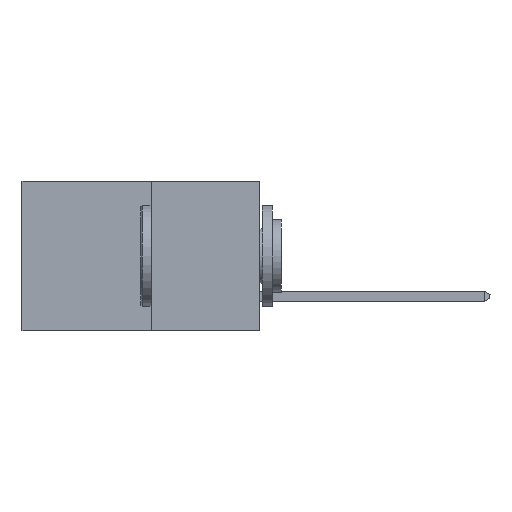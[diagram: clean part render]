
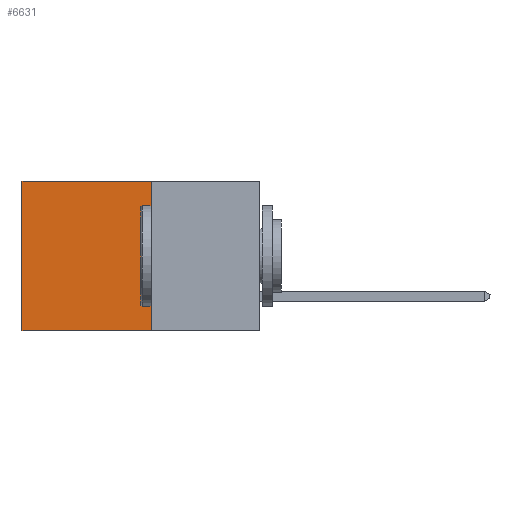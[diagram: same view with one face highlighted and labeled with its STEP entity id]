
A CAD part, left-side view. The second image highlights one B-rep face of the part: STEP entity #6631.
In plain terms, the highlighted planar face has unit normal (-1, 0, 0).
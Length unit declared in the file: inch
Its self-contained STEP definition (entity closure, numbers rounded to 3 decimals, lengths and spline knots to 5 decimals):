
#908 = EDGE_CURVE ( 'NONE', #919, #8544, #1760, .T. ) ;
#919 = VERTEX_POINT ( 'NONE', #2599 ) ;
#1028 = VERTEX_POINT ( 'NONE', #2394 ) ;
#1092 = EDGE_CURVE ( 'NONE', #4921, #1028, #3970, .T. ) ;
#1102 = ORIENTED_EDGE ( 'NONE', *, *, #908, .T. ) ;
#1227 = DIRECTION ( 'NONE',  ( 0., 0., -1. ) ) ;
#1365 = EDGE_CURVE ( 'NONE', #4921, #919, #6006, .T. ) ;
#1760 = LINE ( 'NONE', #6541, #9163 ) ;
#2394 = CARTESIAN_POINT ( 'NONE',  ( 0.277, 0.27, -0.37 ) ) ;
#2599 = CARTESIAN_POINT ( 'NONE',  ( 0.277, 0.59, 0. ) ) ;
#2640 = ORIENTED_EDGE ( 'NONE', *, *, #1365, .T. ) ;
#3188 = CARTESIAN_POINT ( 'NONE',  ( 0.277, 0.27, 0. ) ) ;
#3970 = LINE ( 'NONE', #8597, #5901 ) ;
#4086 = VECTOR ( 'NONE', #6167, 39.37008 ) ;
#4392 = DIRECTION ( 'NONE',  ( 0., 0., -1. ) ) ;
#4405 = DIRECTION ( 'NONE',  ( 1., 0., 0. ) ) ;
#4433 = CARTESIAN_POINT ( 'NONE',  ( 0.277, 0.27, -0.37 ) ) ;
#4444 = PLANE ( 'NONE',  #5884 ) ;
#4632 = DIRECTION ( 'NONE',  ( 0., 0., -1. ) ) ;
#4921 = VERTEX_POINT ( 'NONE', #3188 ) ;
#5164 = CARTESIAN_POINT ( 'NONE',  ( 0.277, 0.59, -0.37 ) ) ;
#5381 = CARTESIAN_POINT ( 'NONE',  ( 0.277, 0.27, -0.37 ) ) ;
#5478 = DIRECTION ( 'NONE',  ( 0., 1., 0. ) ) ;
#5559 = VECTOR ( 'NONE', #5478, 39.37008 ) ;
#5884 = AXIS2_PLACEMENT_3D ( 'NONE', #4433, #4405, #4392 ) ;
#5901 = VECTOR ( 'NONE', #1227, 39.37008 ) ;
#5964 = ORIENTED_EDGE ( 'NONE', *, *, #7662, .F. ) ;
#6006 = LINE ( 'NONE', #6071, #4086 ) ;
#6071 = CARTESIAN_POINT ( 'NONE',  ( 0.277, 0.27, 0. ) ) ;
#6167 = DIRECTION ( 'NONE',  ( 0., 1., 0. ) ) ;
#6541 = CARTESIAN_POINT ( 'NONE',  ( 0.277, 0.59, -0.37 ) ) ;
#6631 = ADVANCED_FACE ( 'NONE', ( #7527 ), #4444, .F. ) ;
#7527 = FACE_OUTER_BOUND ( 'NONE', #7849, .T. ) ;
#7661 = ORIENTED_EDGE ( 'NONE', *, *, #1092, .F. ) ;
#7662 = EDGE_CURVE ( 'NONE', #1028, #8544, #7812, .T. ) ;
#7812 = LINE ( 'NONE', #5381, #5559 ) ;
#7849 = EDGE_LOOP ( 'NONE', ( #1102, #5964, #7661, #2640 ) ) ;
#8544 = VERTEX_POINT ( 'NONE', #5164 ) ;
#8597 = CARTESIAN_POINT ( 'NONE',  ( 0.277, 0.27, -0.37 ) ) ;
#9163 = VECTOR ( 'NONE', #4632, 39.37008 ) ;
